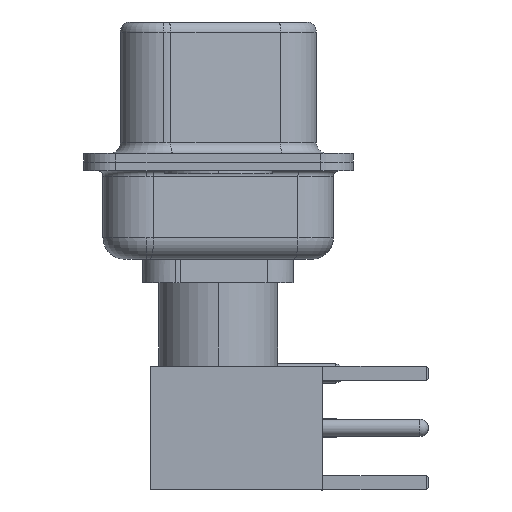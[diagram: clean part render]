
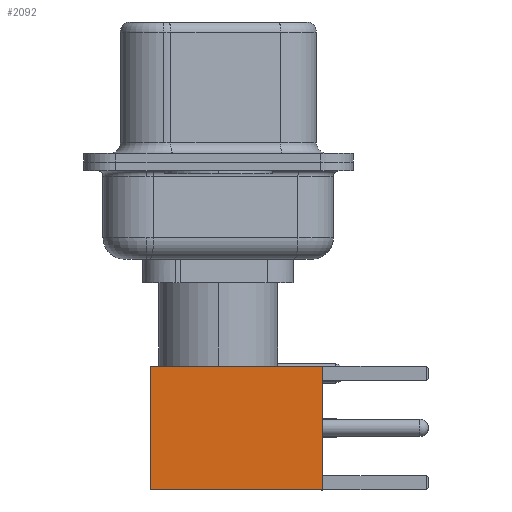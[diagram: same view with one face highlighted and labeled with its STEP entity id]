
A CAD part, left-side view. The second image highlights one B-rep face of the part: STEP entity #2092.
In plain terms, the highlighted face is planar.
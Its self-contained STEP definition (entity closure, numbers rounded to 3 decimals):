
#329 = VECTOR ( 'NONE', #26344, 1000. ) ;
#738 = CARTESIAN_POINT ( 'NONE',  ( 2.875, 2.875, 0. ) ) ;
#1741 = VECTOR ( 'NONE', #7119, 1000. ) ;
#2092 = ADVANCED_FACE ( 'NONE', ( #10393 ), #15233, .T. ) ;
#3614 = ORIENTED_EDGE ( 'NONE', *, *, #25681, .F. ) ;
#3899 = ORIENTED_EDGE ( 'NONE', *, *, #26880, .F. ) ;
#4053 = VECTOR ( 'NONE', #24487, 1000. ) ;
#4163 = CARTESIAN_POINT ( 'NONE',  ( -2.875, 2.875, 0. ) ) ;
#6607 = VERTEX_POINT ( 'NONE', #7665 ) ;
#6691 = VECTOR ( 'NONE', #13657, 1000. ) ;
#6817 = LINE ( 'NONE', #20960, #1741 ) ;
#7119 = DIRECTION ( 'NONE',  ( -1., 0., 0. ) ) ;
#7665 = CARTESIAN_POINT ( 'NONE',  ( -2.875, 2.875, 8. ) ) ;
#10393 = FACE_OUTER_BOUND ( 'NONE', #15818, .T. ) ;
#11587 = AXIS2_PLACEMENT_3D ( 'NONE', #12123, #21604, #24116 ) ;
#12123 = CARTESIAN_POINT ( 'NONE',  ( 2.875, 2.875, 0. ) ) ;
#12283 = VERTEX_POINT ( 'NONE', #14260 ) ;
#13657 = DIRECTION ( 'NONE',  ( 0., 0., -1. ) ) ;
#14260 = CARTESIAN_POINT ( 'NONE',  ( -2.875, 2.875, 0. ) ) ;
#14776 = VERTEX_POINT ( 'NONE', #738 ) ;
#14839 = LINE ( 'NONE', #16852, #329 ) ;
#15233 = PLANE ( 'NONE',  #11587 ) ;
#15528 = LINE ( 'NONE', #4163, #6691 ) ;
#15818 = EDGE_LOOP ( 'NONE', ( #29319, #25955, #3614, #3899 ) ) ;
#16852 = CARTESIAN_POINT ( 'NONE',  ( 0., 2.875, 0. ) ) ;
#20960 = CARTESIAN_POINT ( 'NONE',  ( 0., 2.875, 8. ) ) ;
#21524 = LINE ( 'NONE', #24343, #4053 ) ;
#21604 = DIRECTION ( 'NONE',  ( 0., 1., 0. ) ) ;
#22555 = EDGE_CURVE ( 'NONE', #28336, #14776, #21524, .T. ) ;
#24116 = DIRECTION ( 'NONE',  ( 0., 0., 1. ) ) ;
#24343 = CARTESIAN_POINT ( 'NONE',  ( 2.875, 2.875, 0. ) ) ;
#24487 = DIRECTION ( 'NONE',  ( 0., 0., -1. ) ) ;
#24842 = CARTESIAN_POINT ( 'NONE',  ( 2.875, 2.875, 8. ) ) ;
#25681 = EDGE_CURVE ( 'NONE', #6607, #12283, #15528, .T. ) ;
#25955 = ORIENTED_EDGE ( 'NONE', *, *, #30052, .T. ) ;
#26344 = DIRECTION ( 'NONE',  ( -1., 0., 0. ) ) ;
#26880 = EDGE_CURVE ( 'NONE', #28336, #6607, #6817, .T. ) ;
#28336 = VERTEX_POINT ( 'NONE', #24842 ) ;
#29319 = ORIENTED_EDGE ( 'NONE', *, *, #22555, .T. ) ;
#30052 = EDGE_CURVE ( 'NONE', #14776, #12283, #14839, .T. ) ;
